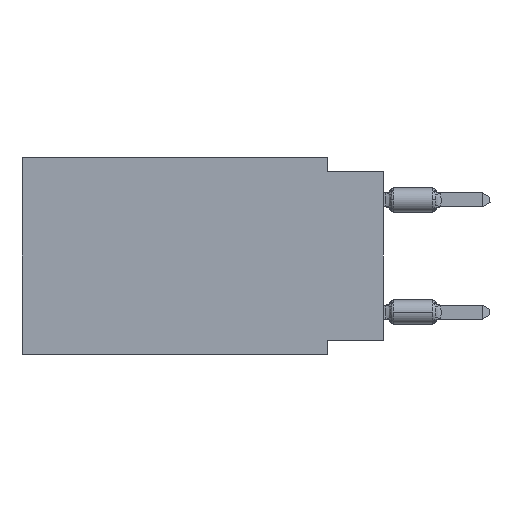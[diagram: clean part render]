
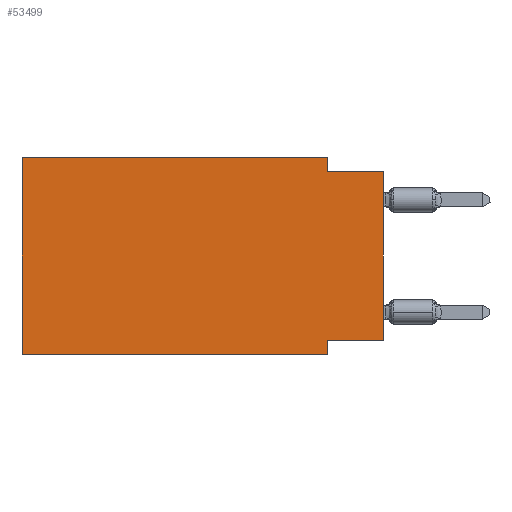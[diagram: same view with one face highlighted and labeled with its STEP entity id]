
A CAD part, left-side view. The second image highlights one B-rep face of the part: STEP entity #53499.
In plain terms, the highlighted planar face has unit normal (-1, 0, 0).
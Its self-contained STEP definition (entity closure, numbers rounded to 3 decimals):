
#474 = CARTESIAN_POINT ( 'NONE',  ( 0., 16.383, -8.89 ) ) ;
#1867 = CARTESIAN_POINT ( 'NONE',  ( 0., 16.383, 0. ) ) ;
#2044 = LINE ( 'NONE', #31533, #48498 ) ;
#2744 = CARTESIAN_POINT ( 'NONE',  ( 0., 2.54, -8.89 ) ) ;
#3721 = DIRECTION ( 'NONE',  ( 1., 0., 0. ) ) ;
#5328 = CARTESIAN_POINT ( 'NONE',  ( 0., 0., -8.255 ) ) ;
#5463 = LINE ( 'NONE', #52235, #41400 ) ;
#5994 = VERTEX_POINT ( 'NONE', #16308 ) ;
#6272 = CARTESIAN_POINT ( 'NONE',  ( 0., 2.54, 0. ) ) ;
#6795 = CARTESIAN_POINT ( 'NONE',  ( 0., 16.383, 0. ) ) ;
#7551 = EDGE_CURVE ( 'NONE', #17785, #8742, #27405, .T. ) ;
#8742 = VERTEX_POINT ( 'NONE', #1867 ) ;
#9662 = ORIENTED_EDGE ( 'NONE', *, *, #47207, .F. ) ;
#10248 = ORIENTED_EDGE ( 'NONE', *, *, #28281, .F. ) ;
#11257 = ORIENTED_EDGE ( 'NONE', *, *, #21851, .F. ) ;
#13000 = ORIENTED_EDGE ( 'NONE', *, *, #42409, .T. ) ;
#15806 = ORIENTED_EDGE ( 'NONE', *, *, #38543, .F. ) ;
#16308 = CARTESIAN_POINT ( 'NONE',  ( 0., 2.54, 0. ) ) ;
#17436 = LINE ( 'NONE', #474, #26503 ) ;
#17785 = VERTEX_POINT ( 'NONE', #53073 ) ;
#17889 = EDGE_LOOP ( 'NONE', ( #13000, #10248, #30223, #11257, #39185, #52842, #15806, #9662 ) ) ;
#18339 = VERTEX_POINT ( 'NONE', #28617 ) ;
#20674 = DIRECTION ( 'NONE',  ( 0., 0., -1. ) ) ;
#21851 = EDGE_CURVE ( 'NONE', #8742, #5994, #5463, .T. ) ;
#24350 = VERTEX_POINT ( 'NONE', #28736 ) ;
#24616 = VERTEX_POINT ( 'NONE', #2744 ) ;
#24620 = CARTESIAN_POINT ( 'NONE',  ( 0., 0., -0.635 ) ) ;
#24884 = DIRECTION ( 'NONE',  ( 0., -1., 0. ) ) ;
#25243 = CARTESIAN_POINT ( 'NONE',  ( 0., 0., -8.255 ) ) ;
#26480 = LINE ( 'NONE', #5328, #40011 ) ;
#26503 = VECTOR ( 'NONE', #30231, 1000. ) ;
#27111 = VECTOR ( 'NONE', #31573, 1000. ) ;
#27405 = LINE ( 'NONE', #6795, #27111 ) ;
#28281 = EDGE_CURVE ( 'NONE', #18339, #24350, #45778, .T. ) ;
#28469 = DIRECTION ( 'NONE',  ( 0., 0., 1. ) ) ;
#28617 = CARTESIAN_POINT ( 'NONE',  ( 0., 2.54, -0.635 ) ) ;
#28736 = CARTESIAN_POINT ( 'NONE',  ( 0., 0., -0.635 ) ) ;
#30223 = ORIENTED_EDGE ( 'NONE', *, *, #45275, .F. ) ;
#30231 = DIRECTION ( 'NONE',  ( 0., -1., 0. ) ) ;
#31533 = CARTESIAN_POINT ( 'NONE',  ( 0., 0., 0. ) ) ;
#31573 = DIRECTION ( 'NONE',  ( 0., 0., 1. ) ) ;
#33201 = PLANE ( 'NONE',  #41796 ) ;
#33487 = LINE ( 'NONE', #54372, #34184 ) ;
#34026 = FACE_OUTER_BOUND ( 'NONE', #17889, .T. ) ;
#34184 = VECTOR ( 'NONE', #41297, 1000. ) ;
#34501 = VECTOR ( 'NONE', #43584, 1000. ) ;
#34822 = DIRECTION ( 'NONE',  ( 0., 1., 0. ) ) ;
#38543 = EDGE_CURVE ( 'NONE', #51234, #24616, #33487, .T. ) ;
#39135 = DIRECTION ( 'NONE',  ( 0., -1., 0. ) ) ;
#39185 = ORIENTED_EDGE ( 'NONE', *, *, #7551, .F. ) ;
#40011 = VECTOR ( 'NONE', #34822, 1000. ) ;
#40694 = CARTESIAN_POINT ( 'NONE',  ( 0., 2.54, -8.255 ) ) ;
#41297 = DIRECTION ( 'NONE',  ( 0., 0., -1. ) ) ;
#41400 = VECTOR ( 'NONE', #39135, 1000. ) ;
#41796 = AXIS2_PLACEMENT_3D ( 'NONE', #46020, #3721, #20674 ) ;
#42409 = EDGE_CURVE ( 'NONE', #43772, #24350, #2044, .T. ) ;
#43584 = DIRECTION ( 'NONE',  ( 0., 0., -1. ) ) ;
#43772 = VERTEX_POINT ( 'NONE', #25243 ) ;
#44411 = LINE ( 'NONE', #6272, #34501 ) ;
#45041 = EDGE_CURVE ( 'NONE', #17785, #24616, #17436, .T. ) ;
#45275 = EDGE_CURVE ( 'NONE', #5994, #18339, #44411, .T. ) ;
#45778 = LINE ( 'NONE', #24620, #46115 ) ;
#46020 = CARTESIAN_POINT ( 'NONE',  ( 0., 16.383, 0. ) ) ;
#46115 = VECTOR ( 'NONE', #24884, 1000. ) ;
#47207 = EDGE_CURVE ( 'NONE', #43772, #51234, #26480, .T. ) ;
#48498 = VECTOR ( 'NONE', #28469, 1000. ) ;
#51234 = VERTEX_POINT ( 'NONE', #40694 ) ;
#52235 = CARTESIAN_POINT ( 'NONE',  ( 0., 16.383, 0. ) ) ;
#52842 = ORIENTED_EDGE ( 'NONE', *, *, #45041, .T. ) ;
#53073 = CARTESIAN_POINT ( 'NONE',  ( 0., 16.383, -8.89 ) ) ;
#53499 = ADVANCED_FACE ( 'NONE', ( #34026 ), #33201, .F. ) ;
#54372 = CARTESIAN_POINT ( 'NONE',  ( 0., 2.54, -8.89 ) ) ;
